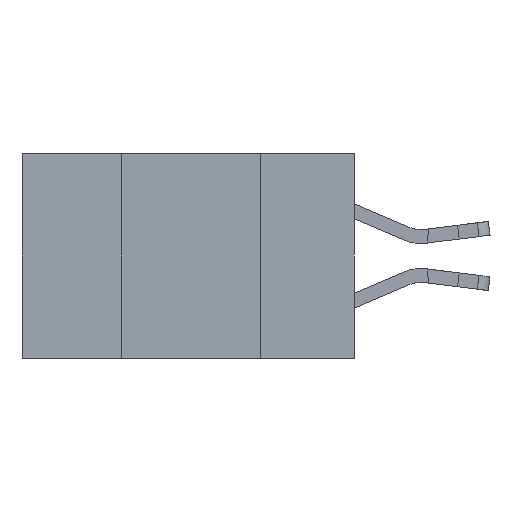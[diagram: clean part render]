
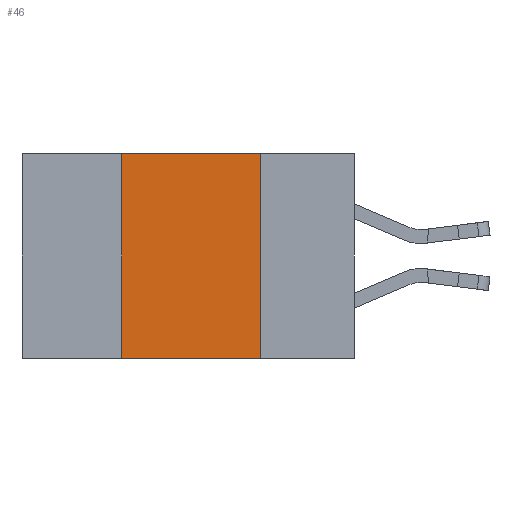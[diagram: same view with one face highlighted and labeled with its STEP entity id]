
A CAD part, left-side view. The second image highlights one B-rep face of the part: STEP entity #46.
In plain terms, the highlighted planar face has unit normal (-1, 0, 0).
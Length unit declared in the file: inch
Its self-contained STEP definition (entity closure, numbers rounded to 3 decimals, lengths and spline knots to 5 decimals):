
#46 = ADVANCED_FACE ( 'NONE', ( #4199 ), #3359, .F. ) ;
#326 = CARTESIAN_POINT ( 'NONE',  ( 0., 0.17, -0.37 ) ) ;
#439 = VERTEX_POINT ( 'NONE', #916 ) ;
#535 = EDGE_LOOP ( 'NONE', ( #658, #9790, #4272, #7578 ) ) ;
#579 = VERTEX_POINT ( 'NONE', #8782 ) ;
#658 = ORIENTED_EDGE ( 'NONE', *, *, #4664, .F. ) ;
#916 = CARTESIAN_POINT ( 'NONE',  ( 0., 0.42, -0.37 ) ) ;
#1126 = DIRECTION ( 'NONE',  ( 0., 0., 1. ) ) ;
#1519 = CARTESIAN_POINT ( 'NONE',  ( 0., 0.17, 0. ) ) ;
#1790 = VERTEX_POINT ( 'NONE', #1519 ) ;
#2149 = LINE ( 'NONE', #7704, #10323 ) ;
#2246 = VERTEX_POINT ( 'NONE', #326 ) ;
#2610 = LINE ( 'NONE', #4627, #9084 ) ;
#3359 = PLANE ( 'NONE',  #5671 ) ;
#3417 = CARTESIAN_POINT ( 'NONE',  ( 0., 0.6, 0. ) ) ;
#3460 = EDGE_CURVE ( 'NONE', #439, #2246, #6662, .T. ) ;
#3461 = EDGE_CURVE ( 'NONE', #579, #1790, #2610, .T. ) ;
#4199 = FACE_OUTER_BOUND ( 'NONE', #535, .T. ) ;
#4272 = ORIENTED_EDGE ( 'NONE', *, *, #5590, .F. ) ;
#4345 = DIRECTION ( 'NONE',  ( 0., -1., 0. ) ) ;
#4627 = CARTESIAN_POINT ( 'NONE',  ( 0., 0.6, 0. ) ) ;
#4664 = EDGE_CURVE ( 'NONE', #1790, #2246, #8092, .T. ) ;
#4993 = DIRECTION ( 'NONE',  ( 0., 0., -1. ) ) ;
#5103 = DIRECTION ( 'NONE',  ( 1., 0., 0. ) ) ;
#5590 = EDGE_CURVE ( 'NONE', #439, #579, #2149, .T. ) ;
#5671 = AXIS2_PLACEMENT_3D ( 'NONE', #3417, #5103, #6627 ) ;
#5682 = CARTESIAN_POINT ( 'NONE',  ( 0., 0.17, -0.37 ) ) ;
#6627 = DIRECTION ( 'NONE',  ( 0., 0., -1. ) ) ;
#6662 = LINE ( 'NONE', #9939, #8593 ) ;
#7535 = VECTOR ( 'NONE', #4993, 39.37008 ) ;
#7578 = ORIENTED_EDGE ( 'NONE', *, *, #3460, .T. ) ;
#7704 = CARTESIAN_POINT ( 'NONE',  ( 0., 0.42, -0.37 ) ) ;
#8092 = LINE ( 'NONE', #5682, #7535 ) ;
#8593 = VECTOR ( 'NONE', #4345, 39.37008 ) ;
#8782 = CARTESIAN_POINT ( 'NONE',  ( 0., 0.42, 0. ) ) ;
#9084 = VECTOR ( 'NONE', #10285, 39.37008 ) ;
#9790 = ORIENTED_EDGE ( 'NONE', *, *, #3461, .F. ) ;
#9939 = CARTESIAN_POINT ( 'NONE',  ( 0., 0.6, -0.37 ) ) ;
#10285 = DIRECTION ( 'NONE',  ( 0., -1., 0. ) ) ;
#10323 = VECTOR ( 'NONE', #1126, 39.37008 ) ;
